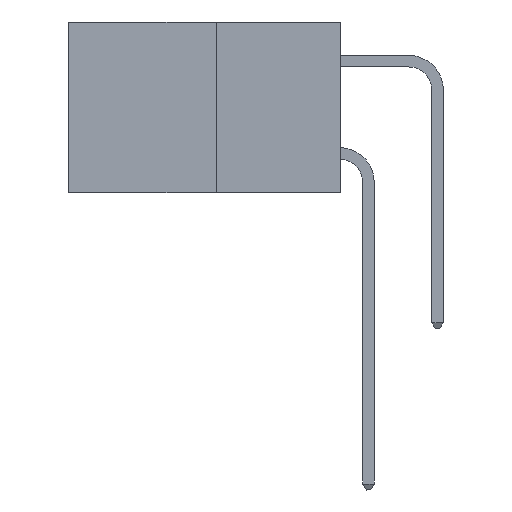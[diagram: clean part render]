
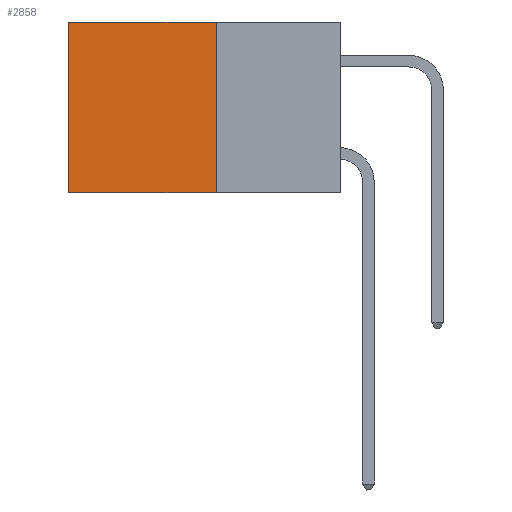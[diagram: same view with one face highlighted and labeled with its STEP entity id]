
A CAD part, left-side view. The second image highlights one B-rep face of the part: STEP entity #2858.
In plain terms, the highlighted planar face has unit normal (-1, 0, 0).
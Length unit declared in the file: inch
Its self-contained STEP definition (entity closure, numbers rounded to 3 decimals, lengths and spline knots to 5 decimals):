
#195 = DIRECTION ( 'NONE',  ( 0., 1., 0. ) ) ;
#394 = ORIENTED_EDGE ( 'NONE', *, *, #7581, .T. ) ;
#581 = FACE_OUTER_BOUND ( 'NONE', #9714, .T. ) ;
#611 = VECTOR ( 'NONE', #1350, 39.37008 ) ;
#1350 = DIRECTION ( 'NONE',  ( 0., 0., -1. ) ) ;
#1354 = CARTESIAN_POINT ( 'NONE',  ( 0.277, 0.27, -0.37 ) ) ;
#2469 = ORIENTED_EDGE ( 'NONE', *, *, #4036, .F. ) ;
#2858 = ADVANCED_FACE ( 'NONE', ( #581 ), #6317, .F. ) ;
#3092 = CARTESIAN_POINT ( 'NONE',  ( 0.277, 0.27, 0. ) ) ;
#3360 = VERTEX_POINT ( 'NONE', #4891 ) ;
#3531 = CARTESIAN_POINT ( 'NONE',  ( 0.277, 0.27, -0.37 ) ) ;
#3540 = DIRECTION ( 'NONE',  ( 0., 1., 0. ) ) ;
#3735 = CARTESIAN_POINT ( 'NONE',  ( 0.277, 0.59, -0.37 ) ) ;
#4036 = EDGE_CURVE ( 'NONE', #9010, #3360, #6321, .T. ) ;
#4163 = VECTOR ( 'NONE', #4683, 39.37008 ) ;
#4683 = DIRECTION ( 'NONE',  ( 0., 0., -1. ) ) ;
#4891 = CARTESIAN_POINT ( 'NONE',  ( 0.277, 0.59, -0.37 ) ) ;
#5509 = EDGE_CURVE ( 'NONE', #12068, #9010, #5680, .T. ) ;
#5590 = DIRECTION ( 'NONE',  ( 0., 0., -1. ) ) ;
#5603 = DIRECTION ( 'NONE',  ( 1., 0., 0. ) ) ;
#5647 = CARTESIAN_POINT ( 'NONE',  ( 0.277, 0.27, -0.37 ) ) ;
#5680 = LINE ( 'NONE', #1354, #611 ) ;
#6317 = PLANE ( 'NONE',  #8526 ) ;
#6321 = LINE ( 'NONE', #3531, #10798 ) ;
#7144 = CARTESIAN_POINT ( 'NONE',  ( 0.277, 0.59, 0. ) ) ;
#7581 = EDGE_CURVE ( 'NONE', #8129, #3360, #11310, .T. ) ;
#8046 = ORIENTED_EDGE ( 'NONE', *, *, #5509, .F. ) ;
#8121 = EDGE_CURVE ( 'NONE', #12068, #8129, #11789, .T. ) ;
#8129 = VERTEX_POINT ( 'NONE', #7144 ) ;
#8526 = AXIS2_PLACEMENT_3D ( 'NONE', #5647, #5603, #5590 ) ;
#9010 = VERTEX_POINT ( 'NONE', #10906 ) ;
#9714 = EDGE_LOOP ( 'NONE', ( #394, #2469, #8046, #10443 ) ) ;
#10443 = ORIENTED_EDGE ( 'NONE', *, *, #8121, .T. ) ;
#10798 = VECTOR ( 'NONE', #3540, 39.37008 ) ;
#10906 = CARTESIAN_POINT ( 'NONE',  ( 0.277, 0.27, -0.37 ) ) ;
#11310 = LINE ( 'NONE', #3735, #4163 ) ;
#11483 = CARTESIAN_POINT ( 'NONE',  ( 0.277, 0.27, 0. ) ) ;
#11547 = VECTOR ( 'NONE', #195, 39.37008 ) ;
#11789 = LINE ( 'NONE', #11483, #11547 ) ;
#12068 = VERTEX_POINT ( 'NONE', #3092 ) ;
